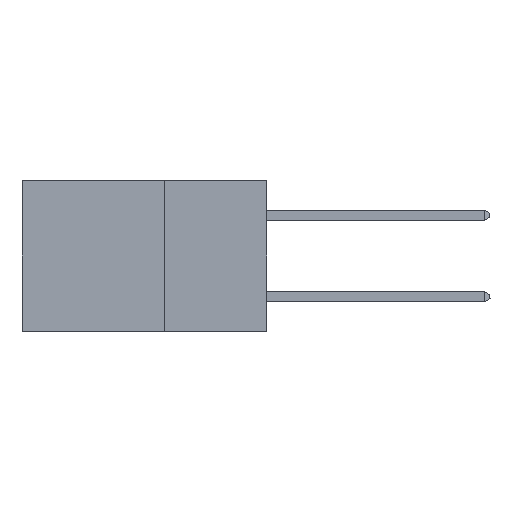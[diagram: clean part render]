
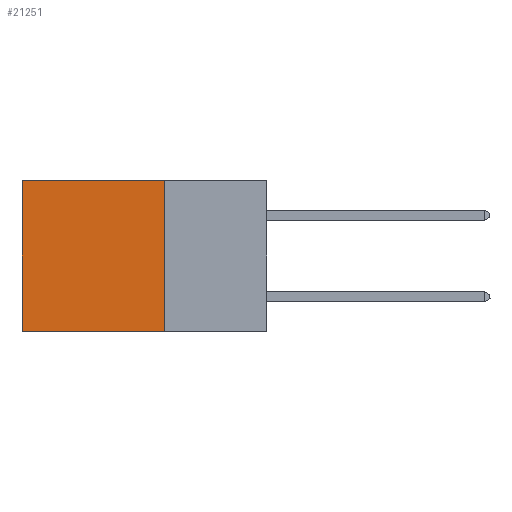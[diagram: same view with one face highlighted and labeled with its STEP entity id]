
A CAD part, left-side view. The second image highlights one B-rep face of the part: STEP entity #21251.
In plain terms, the highlighted planar face has unit normal (-1, 0, 0).
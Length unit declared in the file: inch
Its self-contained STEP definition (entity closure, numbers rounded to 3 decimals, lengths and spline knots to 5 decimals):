
#335 = VERTEX_POINT ( 'NONE', #9776 ) ;
#772 = VECTOR ( 'NONE', #17882, 39.37008 ) ;
#1088 = LINE ( 'NONE', #26513, #772 ) ;
#1778 = VERTEX_POINT ( 'NONE', #3959 ) ;
#2795 = EDGE_CURVE ( 'NONE', #1778, #14837, #20838, .T. ) ;
#3959 = CARTESIAN_POINT ( 'NONE',  ( 0.2875, 0.6, 0. ) ) ;
#4382 = ORIENTED_EDGE ( 'NONE', *, *, #2795, .T. ) ;
#4852 = CARTESIAN_POINT ( 'NONE',  ( 0.2875, 0.6, 0. ) ) ;
#7169 = LINE ( 'NONE', #27902, #9862 ) ;
#8205 = DIRECTION ( 'NONE',  ( 0., 0., -1. ) ) ;
#8419 = FACE_OUTER_BOUND ( 'NONE', #9588, .T. ) ;
#9400 = DIRECTION ( 'NONE',  ( 1., 0., 0. ) ) ;
#9588 = EDGE_LOOP ( 'NONE', ( #4382, #14271, #24131, #25680 ) ) ;
#9776 = CARTESIAN_POINT ( 'NONE',  ( 0.2875, 0.25, -0.37 ) ) ;
#9862 = VECTOR ( 'NONE', #17383, 39.37008 ) ;
#9879 = EDGE_CURVE ( 'NONE', #19385, #335, #7169, .T. ) ;
#11591 = DIRECTION ( 'NONE',  ( 0., 0., -1. ) ) ;
#11722 = EDGE_CURVE ( 'NONE', #19385, #1778, #19498, .T. ) ;
#12424 = VECTOR ( 'NONE', #18001, 39.37008 ) ;
#13263 = CARTESIAN_POINT ( 'NONE',  ( 0.2875, 0.25, 0. ) ) ;
#14105 = VECTOR ( 'NONE', #8205, 39.37008 ) ;
#14271 = ORIENTED_EDGE ( 'NONE', *, *, #15263, .F. ) ;
#14837 = VERTEX_POINT ( 'NONE', #21271 ) ;
#15263 = EDGE_CURVE ( 'NONE', #335, #14837, #1088, .T. ) ;
#15838 = CARTESIAN_POINT ( 'NONE',  ( 0.2875, 0.25, 0. ) ) ;
#15908 = PLANE ( 'NONE',  #26131 ) ;
#17383 = DIRECTION ( 'NONE',  ( 0., 0., -1. ) ) ;
#17882 = DIRECTION ( 'NONE',  ( 0., 1., 0. ) ) ;
#18001 = DIRECTION ( 'NONE',  ( 0., 1., 0. ) ) ;
#19385 = VERTEX_POINT ( 'NONE', #24393 ) ;
#19498 = LINE ( 'NONE', #15838, #12424 ) ;
#20838 = LINE ( 'NONE', #4852, #14105 ) ;
#21251 = ADVANCED_FACE ( 'NONE', ( #8419 ), #15908, .F. ) ;
#21271 = CARTESIAN_POINT ( 'NONE',  ( 0.2875, 0.6, -0.37 ) ) ;
#24131 = ORIENTED_EDGE ( 'NONE', *, *, #9879, .F. ) ;
#24393 = CARTESIAN_POINT ( 'NONE',  ( 0.2875, 0.25, 0. ) ) ;
#25680 = ORIENTED_EDGE ( 'NONE', *, *, #11722, .T. ) ;
#26131 = AXIS2_PLACEMENT_3D ( 'NONE', #13263, #9400, #11591 ) ;
#26513 = CARTESIAN_POINT ( 'NONE',  ( 0.2875, 0.25, -0.37 ) ) ;
#27902 = CARTESIAN_POINT ( 'NONE',  ( 0.2875, 0.25, 0. ) ) ;
